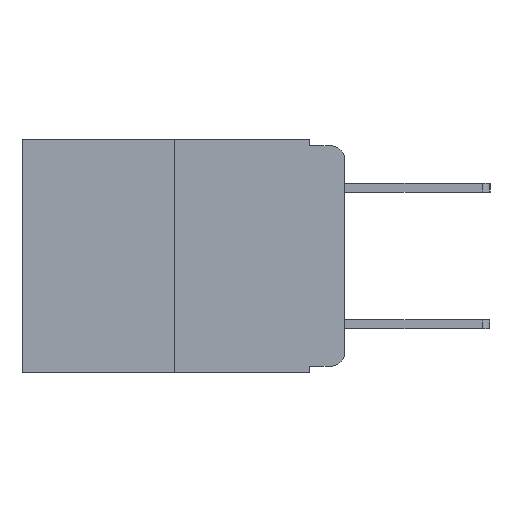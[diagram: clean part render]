
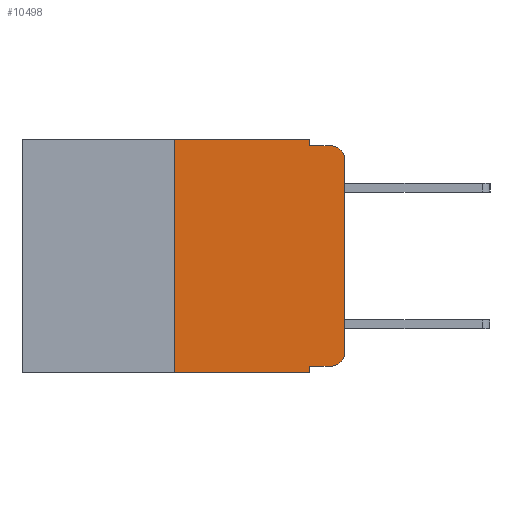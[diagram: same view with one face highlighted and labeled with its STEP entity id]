
A CAD part, left-side view. The second image highlights one B-rep face of the part: STEP entity #10498.
In plain terms, the highlighted planar face has unit normal (-1, 0, 0).
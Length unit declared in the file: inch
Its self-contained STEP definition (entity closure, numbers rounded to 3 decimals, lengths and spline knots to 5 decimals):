
#477 = EDGE_LOOP ( 'NONE', ( #14884, #14060, #4849, #5698, #16046, #17919, #3990, #15636, #5211, #2798 ) ) ;
#804 = CARTESIAN_POINT ( 'NONE',  ( 0., 0.02, -0.01 ) ) ;
#1012 = VECTOR ( 'NONE', #5288, 39.37008 ) ;
#1065 = LINE ( 'NONE', #15700, #8729 ) ;
#1316 = CARTESIAN_POINT ( 'NONE',  ( 0., 0.02, -0.313 ) ) ;
#1477 = CARTESIAN_POINT ( 'NONE',  ( 0., 0.051, -0.01 ) ) ;
#2021 = CIRCLE ( 'NONE', #17192, 0.02 ) ;
#2798 = ORIENTED_EDGE ( 'NONE', *, *, #16380, .T. ) ;
#2909 = DIRECTION ( 'NONE',  ( 0., 0., -1. ) ) ;
#3112 = EDGE_CURVE ( 'NONE', #9460, #11982, #4141, .T. ) ;
#3622 = DIRECTION ( 'NONE',  ( 0., 0., 1. ) ) ;
#3648 = CARTESIAN_POINT ( 'NONE',  ( 0., 0.25, 0. ) ) ;
#3812 = DIRECTION ( 'NONE',  ( 0., -1., 0. ) ) ;
#3914 = LINE ( 'NONE', #13211, #10327 ) ;
#3990 = ORIENTED_EDGE ( 'NONE', *, *, #3112, .T. ) ;
#4141 = LINE ( 'NONE', #4428, #11759 ) ;
#4428 = CARTESIAN_POINT ( 'NONE',  ( 0., 0.473, -0.343 ) ) ;
#4587 = VECTOR ( 'NONE', #3622, 39.37008 ) ;
#4740 = DIRECTION ( 'NONE',  ( 0., 0., -1. ) ) ;
#4849 = ORIENTED_EDGE ( 'NONE', *, *, #9328, .F. ) ;
#5211 = ORIENTED_EDGE ( 'NONE', *, *, #12802, .T. ) ;
#5288 = DIRECTION ( 'NONE',  ( 0., 0., -1. ) ) ;
#5567 = DIRECTION ( 'NONE',  ( -1., 0., 0. ) ) ;
#5698 = ORIENTED_EDGE ( 'NONE', *, *, #9564, .F. ) ;
#5925 = CARTESIAN_POINT ( 'NONE',  ( 0., 0.051, -0.343 ) ) ;
#6216 = DIRECTION ( 'NONE',  ( 0., -1., 0. ) ) ;
#7219 = EDGE_CURVE ( 'NONE', #15270, #11982, #16714, .T. ) ;
#7408 = VECTOR ( 'NONE', #12264, 39.37008 ) ;
#7877 = LINE ( 'NONE', #3648, #7408 ) ;
#8245 = CIRCLE ( 'NONE', #17727, 0.02 ) ;
#8355 = LINE ( 'NONE', #1477, #15165 ) ;
#8395 = CARTESIAN_POINT ( 'NONE',  ( 0., 0.473, 0. ) ) ;
#8729 = VECTOR ( 'NONE', #17050, 39.37008 ) ;
#8968 = VERTEX_POINT ( 'NONE', #16147 ) ;
#8991 = LINE ( 'NONE', #13564, #4587 ) ;
#9328 = EDGE_CURVE ( 'NONE', #8968, #12398, #8355, .T. ) ;
#9419 = CARTESIAN_POINT ( 'NONE',  ( 0., 0.25, -0.343 ) ) ;
#9460 = VERTEX_POINT ( 'NONE', #9419 ) ;
#9564 = EDGE_CURVE ( 'NONE', #18423, #8968, #3914, .T. ) ;
#9639 = CARTESIAN_POINT ( 'NONE',  ( 0., 0.051, 0. ) ) ;
#9802 = DIRECTION ( 'NONE',  ( 0., 0., -1. ) ) ;
#10138 = VERTEX_POINT ( 'NONE', #16994 ) ;
#10187 = CARTESIAN_POINT ( 'NONE',  ( 0., 0.25, 0. ) ) ;
#10327 = VECTOR ( 'NONE', #4740, 39.37008 ) ;
#10425 = EDGE_CURVE ( 'NONE', #9460, #16325, #7877, .T. ) ;
#10498 = ADVANCED_FACE ( 'NONE', ( #16593 ), #15172, .F. ) ;
#11015 = EDGE_CURVE ( 'NONE', #12644, #10138, #8991, .T. ) ;
#11497 = VERTEX_POINT ( 'NONE', #13147 ) ;
#11504 = CARTESIAN_POINT ( 'NONE',  ( 0., 0., -0.313 ) ) ;
#11640 = DIRECTION ( 'NONE',  ( -1., 0., 0. ) ) ;
#11658 = CARTESIAN_POINT ( 'NONE',  ( 0., 0.051, -0.333 ) ) ;
#11759 = VECTOR ( 'NONE', #3812, 39.37008 ) ;
#11785 = CARTESIAN_POINT ( 'NONE',  ( 0., 0.051, -0.333 ) ) ;
#11982 = VERTEX_POINT ( 'NONE', #5925 ) ;
#12264 = DIRECTION ( 'NONE',  ( 0., 0., 1. ) ) ;
#12317 = CARTESIAN_POINT ( 'NONE',  ( 0., 0.051, 0. ) ) ;
#12398 = VERTEX_POINT ( 'NONE', #804 ) ;
#12520 = LINE ( 'NONE', #11785, #16095 ) ;
#12644 = VERTEX_POINT ( 'NONE', #11504 ) ;
#12802 = EDGE_CURVE ( 'NONE', #15270, #11497, #12520, .T. ) ;
#13147 = CARTESIAN_POINT ( 'NONE',  ( 0., 0.02, -0.333 ) ) ;
#13167 = DIRECTION ( 'NONE',  ( 0., -1., 0. ) ) ;
#13211 = CARTESIAN_POINT ( 'NONE',  ( 0., 0.051, 0. ) ) ;
#13564 = CARTESIAN_POINT ( 'NONE',  ( 0., 0., 0. ) ) ;
#13951 = CARTESIAN_POINT ( 'NONE',  ( 0., 0.02, -0.03 ) ) ;
#14060 = ORIENTED_EDGE ( 'NONE', *, *, #16886, .T. ) ;
#14393 = AXIS2_PLACEMENT_3D ( 'NONE', #8395, #17822, #9802 ) ;
#14884 = ORIENTED_EDGE ( 'NONE', *, *, #11015, .T. ) ;
#15165 = VECTOR ( 'NONE', #6216, 39.37008 ) ;
#15172 = PLANE ( 'NONE',  #14393 ) ;
#15270 = VERTEX_POINT ( 'NONE', #11658 ) ;
#15290 = DIRECTION ( 'NONE',  ( 0., 0., -1. ) ) ;
#15636 = ORIENTED_EDGE ( 'NONE', *, *, #7219, .F. ) ;
#15700 = CARTESIAN_POINT ( 'NONE',  ( 0., 0.473, 0. ) ) ;
#16046 = ORIENTED_EDGE ( 'NONE', *, *, #16415, .F. ) ;
#16095 = VECTOR ( 'NONE', #13167, 39.37008 ) ;
#16147 = CARTESIAN_POINT ( 'NONE',  ( 0., 0.051, -0.01 ) ) ;
#16325 = VERTEX_POINT ( 'NONE', #10187 ) ;
#16380 = EDGE_CURVE ( 'NONE', #11497, #12644, #2021, .T. ) ;
#16415 = EDGE_CURVE ( 'NONE', #16325, #18423, #1065, .T. ) ;
#16593 = FACE_OUTER_BOUND ( 'NONE', #477, .T. ) ;
#16714 = LINE ( 'NONE', #12317, #1012 ) ;
#16886 = EDGE_CURVE ( 'NONE', #10138, #12398, #8245, .T. ) ;
#16994 = CARTESIAN_POINT ( 'NONE',  ( 0., 0., -0.03 ) ) ;
#17050 = DIRECTION ( 'NONE',  ( 0., -1., 0. ) ) ;
#17192 = AXIS2_PLACEMENT_3D ( 'NONE', #1316, #11640, #2909 ) ;
#17727 = AXIS2_PLACEMENT_3D ( 'NONE', #13951, #5567, #15290 ) ;
#17822 = DIRECTION ( 'NONE',  ( 1., 0., 0. ) ) ;
#17919 = ORIENTED_EDGE ( 'NONE', *, *, #10425, .F. ) ;
#18423 = VERTEX_POINT ( 'NONE', #9639 ) ;
